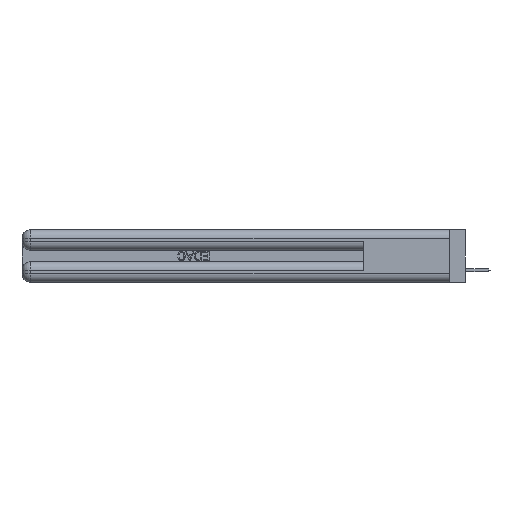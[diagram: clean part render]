
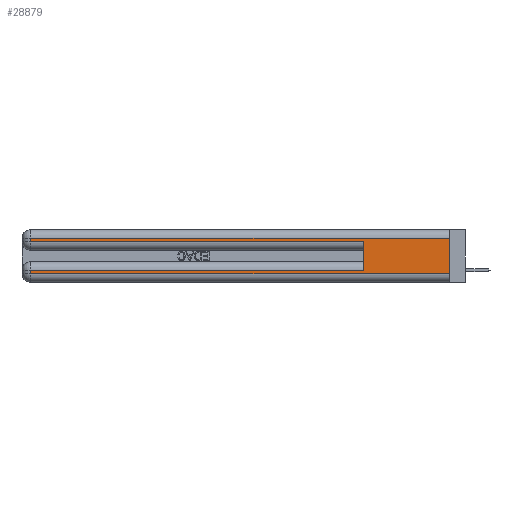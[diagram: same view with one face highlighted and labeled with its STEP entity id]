
A CAD part, left-side view. The second image highlights one B-rep face of the part: STEP entity #28879.
In plain terms, the highlighted planar face has unit normal (-1, 0, 0).
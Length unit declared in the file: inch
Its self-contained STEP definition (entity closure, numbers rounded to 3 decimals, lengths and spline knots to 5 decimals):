
#270 = EDGE_CURVE ( 'NONE', #18772, #10001, #10814, .T. ) ;
#806 = VECTOR ( 'NONE', #32518, 39.37008 ) ;
#1588 = DIRECTION ( 'NONE',  ( 0., 0., 1. ) ) ;
#2045 = CARTESIAN_POINT ( 'NONE',  ( 0., 2.94, 0.37 ) ) ;
#2564 = EDGE_CURVE ( 'NONE', #31144, #18772, #24867, .T. ) ;
#4155 = CARTESIAN_POINT ( 'NONE',  ( 0., 0., 0.31 ) ) ;
#5302 = VECTOR ( 'NONE', #21539, 39.37008 ) ;
#6523 = VECTOR ( 'NONE', #31657, 39.37008 ) ;
#7175 = CARTESIAN_POINT ( 'NONE',  ( 0., 0., 0.06 ) ) ;
#7297 = DIRECTION ( 'NONE',  ( 0., 0., -1. ) ) ;
#7927 = EDGE_CURVE ( 'NONE', #10001, #12875, #20863, .T. ) ;
#9624 = LINE ( 'NONE', #18598, #6523 ) ;
#10001 = VERTEX_POINT ( 'NONE', #20477 ) ;
#10464 = CARTESIAN_POINT ( 'NONE',  ( 0., 0., 0.37 ) ) ;
#10814 = LINE ( 'NONE', #2045, #5302 ) ;
#11075 = ORIENTED_EDGE ( 'NONE', *, *, #35768, .F. ) ;
#12605 = VECTOR ( 'NONE', #13847, 39.37008 ) ;
#12875 = VERTEX_POINT ( 'NONE', #30294 ) ;
#13012 = LINE ( 'NONE', #36052, #806 ) ;
#13143 = VECTOR ( 'NONE', #1588, 39.37008 ) ;
#13342 = CARTESIAN_POINT ( 'NONE',  ( 0., 0., 0.285 ) ) ;
#13790 = ORIENTED_EDGE ( 'NONE', *, *, #270, .T. ) ;
#13847 = DIRECTION ( 'NONE',  ( 0., -1., 0. ) ) ;
#14130 = EDGE_LOOP ( 'NONE', ( #11075, #41067, #13790, #31413, #33415, #27811, #38926, #22932 ) ) ;
#17785 = CARTESIAN_POINT ( 'NONE',  ( 0., 0., 0.37 ) ) ;
#18598 = CARTESIAN_POINT ( 'NONE',  ( 0., 0., 0.085 ) ) ;
#18772 = VERTEX_POINT ( 'NONE', #26369 ) ;
#20096 = EDGE_CURVE ( 'NONE', #28741, #12875, #25311, .T. ) ;
#20162 = CARTESIAN_POINT ( 'NONE',  ( 0., 0., 0.06 ) ) ;
#20393 = VERTEX_POINT ( 'NONE', #27952 ) ;
#20477 = CARTESIAN_POINT ( 'NONE',  ( 0., 2.94, 0.285 ) ) ;
#20863 = LINE ( 'NONE', #13342, #34068 ) ;
#21539 = DIRECTION ( 'NONE',  ( 0., 0., -1. ) ) ;
#21648 = DIRECTION ( 'NONE',  ( 0., 0., -1. ) ) ;
#22873 = EDGE_CURVE ( 'NONE', #28741, #29551, #9624, .T. ) ;
#22932 = ORIENTED_EDGE ( 'NONE', *, *, #23701, .T. ) ;
#23701 = EDGE_CURVE ( 'NONE', #20393, #39210, #32349, .T. ) ;
#24377 = EDGE_CURVE ( 'NONE', #29551, #20393, #13012, .T. ) ;
#24867 = LINE ( 'NONE', #39547, #27964 ) ;
#25311 = LINE ( 'NONE', #40403, #13143 ) ;
#26369 = CARTESIAN_POINT ( 'NONE',  ( 0., 2.94, 0.31 ) ) ;
#27337 = CARTESIAN_POINT ( 'NONE',  ( 0., 0.6, 0.085 ) ) ;
#27811 = ORIENTED_EDGE ( 'NONE', *, *, #22873, .T. ) ;
#27908 = PLANE ( 'NONE',  #28202 ) ;
#27952 = CARTESIAN_POINT ( 'NONE',  ( 0., 2.94, 0.06 ) ) ;
#27964 = VECTOR ( 'NONE', #32853, 39.37008 ) ;
#28202 = AXIS2_PLACEMENT_3D ( 'NONE', #17785, #31151, #21648 ) ;
#28741 = VERTEX_POINT ( 'NONE', #27337 ) ;
#28829 = CARTESIAN_POINT ( 'NONE',  ( 0., 2.94, 0.085 ) ) ;
#28879 = ADVANCED_FACE ( 'NONE', ( #36823 ), #27908, .F. ) ;
#29551 = VERTEX_POINT ( 'NONE', #28829 ) ;
#30294 = CARTESIAN_POINT ( 'NONE',  ( 0., 0.6, 0.285 ) ) ;
#31144 = VERTEX_POINT ( 'NONE', #4155 ) ;
#31151 = DIRECTION ( 'NONE',  ( 1., 0., 0. ) ) ;
#31413 = ORIENTED_EDGE ( 'NONE', *, *, #7927, .T. ) ;
#31657 = DIRECTION ( 'NONE',  ( 0., 1., 0. ) ) ;
#32349 = LINE ( 'NONE', #7175, #12605 ) ;
#32518 = DIRECTION ( 'NONE',  ( 0., 0., -1. ) ) ;
#32853 = DIRECTION ( 'NONE',  ( 0., 1., 0. ) ) ;
#33415 = ORIENTED_EDGE ( 'NONE', *, *, #20096, .F. ) ;
#34068 = VECTOR ( 'NONE', #40844, 39.37008 ) ;
#34151 = VECTOR ( 'NONE', #7297, 39.37008 ) ;
#35768 = EDGE_CURVE ( 'NONE', #31144, #39210, #36156, .T. ) ;
#36052 = CARTESIAN_POINT ( 'NONE',  ( 0., 2.94, 0.37 ) ) ;
#36156 = LINE ( 'NONE', #10464, #34151 ) ;
#36823 = FACE_OUTER_BOUND ( 'NONE', #14130, .T. ) ;
#38926 = ORIENTED_EDGE ( 'NONE', *, *, #24377, .T. ) ;
#39210 = VERTEX_POINT ( 'NONE', #20162 ) ;
#39547 = CARTESIAN_POINT ( 'NONE',  ( 0., 0., 0.31 ) ) ;
#40403 = CARTESIAN_POINT ( 'NONE',  ( 0., 0.6, 0.145 ) ) ;
#40844 = DIRECTION ( 'NONE',  ( 0., -1., 0. ) ) ;
#41067 = ORIENTED_EDGE ( 'NONE', *, *, #2564, .T. ) ;
